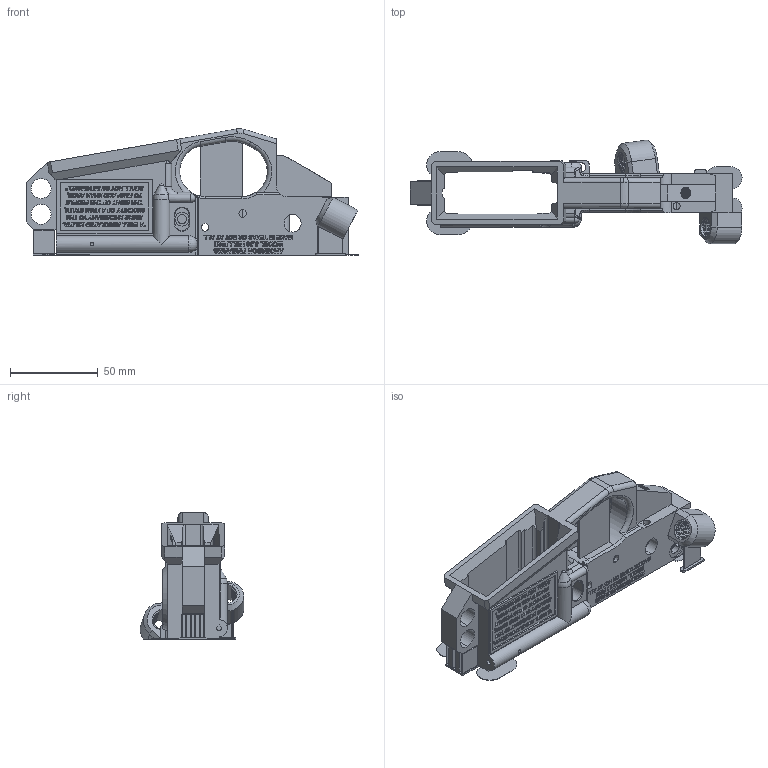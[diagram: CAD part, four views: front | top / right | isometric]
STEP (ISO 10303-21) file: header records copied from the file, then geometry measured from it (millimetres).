
FILE_DESCRIPTION (( 'STEP AP203' ), '1' );
FILE_NAME ('AF-HF-LR-PRT-001-STEP.STEP', '2020-11-04T14:27:32', ( '' ), ( '' ), 'SwSTEP 2.0', 'SolidWorks 2018', '' );
FILE_SCHEMA (( 'CONFIG_CONTROL_DESIGN' ));
Length unit declared in the file: inch
Products named in the file (1): AF-HF-LR-PRT-001-STEP
Bounding box: 189.67 x 59.15 x 72.31 mm (x, y, z)
Volume: 103055.7 mm3; surface area: 75756.6 mm2
Topology: 5 solids, 5 shells, 3331 faces, 9116 edges, 6035 vertices
Faces by surface type: plane 2223, bspline 768, cylinder 295, torus 22, cone 19, sphere 4
Entity records: 186029 total; most frequent: CARTESIAN_POINT 107666, ORIENTED_EDGE 18220, DIRECTION 12783, EDGE_CURVE 9110, LINE 6677, VECTOR 6677, VERTEX_POINT 6034, EDGE_LOOP 3622
